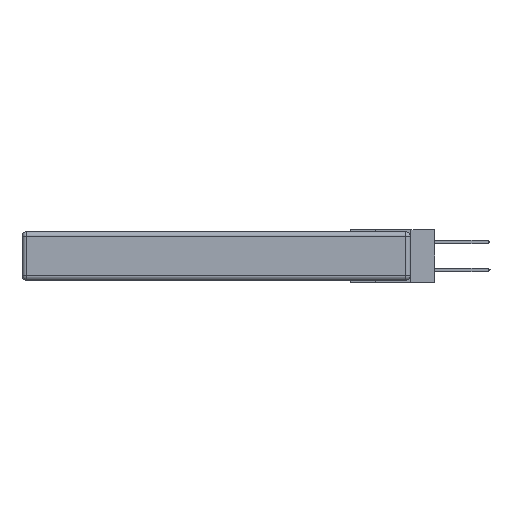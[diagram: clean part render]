
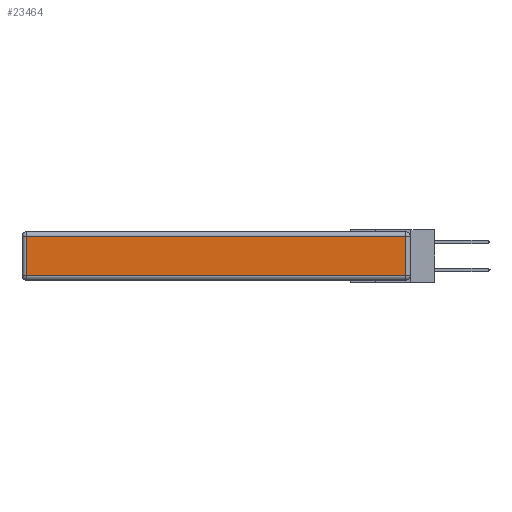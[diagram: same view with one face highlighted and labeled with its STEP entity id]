
A CAD part, left-side view. The second image highlights one B-rep face of the part: STEP entity #23464.
In plain terms, the highlighted planar face has unit normal (-1, 0, 0).
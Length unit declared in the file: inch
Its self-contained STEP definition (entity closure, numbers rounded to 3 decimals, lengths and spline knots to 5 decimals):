
#49 = ORIENTED_EDGE ( 'NONE', *, *, #23052, .T. ) ;
#795 = VERTEX_POINT ( 'NONE', #10617 ) ;
#1638 = CARTESIAN_POINT ( 'NONE',  ( 0., 0.03, -0.313 ) ) ;
#1765 = CARTESIAN_POINT ( 'NONE',  ( 0., 2.72, -0.03 ) ) ;
#4203 = DIRECTION ( 'NONE',  ( 0., 0., 1. ) ) ;
#4391 = LINE ( 'NONE', #5445, #14661 ) ;
#5445 = CARTESIAN_POINT ( 'NONE',  ( 0., 0.03, -0.343 ) ) ;
#6204 = CARTESIAN_POINT ( 'NONE',  ( 0., 2.72, -0.343 ) ) ;
#8045 = AXIS2_PLACEMENT_3D ( 'NONE', #14919, #19421, #4203 ) ;
#10617 = CARTESIAN_POINT ( 'NONE',  ( 0., 2.72, -0.313 ) ) ;
#11869 = ORIENTED_EDGE ( 'NONE', *, *, #18947, .T. ) ;
#12348 = DIRECTION ( 'NONE',  ( 0., -1., 0. ) ) ;
#13748 = ORIENTED_EDGE ( 'NONE', *, *, #20301, .T. ) ;
#14489 = VECTOR ( 'NONE', #12348, 39.37008 ) ;
#14661 = VECTOR ( 'NONE', #17676, 39.37008 ) ;
#14919 = CARTESIAN_POINT ( 'NONE',  ( 0., 0., -0.343 ) ) ;
#15279 = CARTESIAN_POINT ( 'NONE',  ( 0., 2.75, -0.03 ) ) ;
#17493 = ORIENTED_EDGE ( 'NONE', *, *, #25521, .T. ) ;
#17676 = DIRECTION ( 'NONE',  ( 0., 0., 1. ) ) ;
#17946 = EDGE_LOOP ( 'NONE', ( #13748, #17493, #11869, #49 ) ) ;
#18947 = EDGE_CURVE ( 'NONE', #22115, #22811, #25511, .T. ) ;
#19421 = DIRECTION ( 'NONE',  ( -1., 0., 0. ) ) ;
#19716 = VECTOR ( 'NONE', #23994, 39.37008 ) ;
#20301 = EDGE_CURVE ( 'NONE', #795, #28220, #24056, .T. ) ;
#21140 = DIRECTION ( 'NONE',  ( 0., 0., -1. ) ) ;
#22115 = VERTEX_POINT ( 'NONE', #24127 ) ;
#22291 = FACE_OUTER_BOUND ( 'NONE', #17946, .T. ) ;
#22811 = VERTEX_POINT ( 'NONE', #1765 ) ;
#23052 = EDGE_CURVE ( 'NONE', #22811, #795, #27373, .T. ) ;
#23103 = CARTESIAN_POINT ( 'NONE',  ( 0., 0., -0.313 ) ) ;
#23464 = ADVANCED_FACE ( 'NONE', ( #22291 ), #23649, .T. ) ;
#23649 = PLANE ( 'NONE',  #8045 ) ;
#23994 = DIRECTION ( 'NONE',  ( 0., 1., 0. ) ) ;
#24056 = LINE ( 'NONE', #23103, #14489 ) ;
#24127 = CARTESIAN_POINT ( 'NONE',  ( 0., 0.03, -0.03 ) ) ;
#25308 = VECTOR ( 'NONE', #21140, 39.37008 ) ;
#25511 = LINE ( 'NONE', #15279, #19716 ) ;
#25521 = EDGE_CURVE ( 'NONE', #28220, #22115, #4391, .T. ) ;
#27373 = LINE ( 'NONE', #6204, #25308 ) ;
#28220 = VERTEX_POINT ( 'NONE', #1638 ) ;
